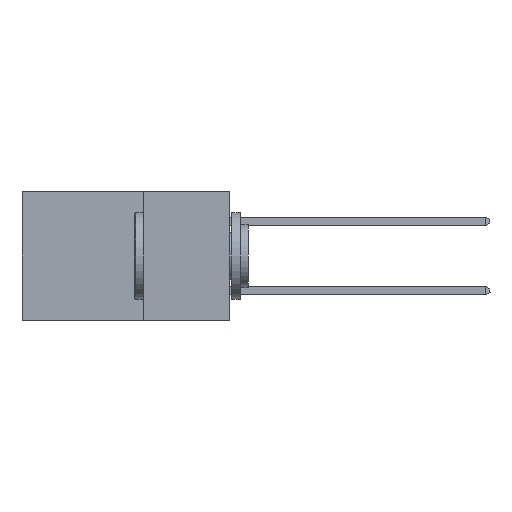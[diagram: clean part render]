
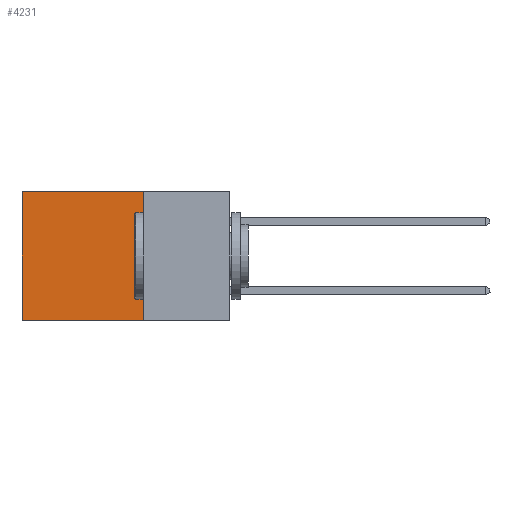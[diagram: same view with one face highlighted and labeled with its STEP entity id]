
A CAD part, left-side view. The second image highlights one B-rep face of the part: STEP entity #4231.
In plain terms, the highlighted planar face has unit normal (-1, 0, 0).
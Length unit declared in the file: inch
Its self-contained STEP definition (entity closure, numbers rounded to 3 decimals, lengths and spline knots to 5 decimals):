
#115 = ORIENTED_EDGE ( 'NONE', *, *, #20439, .F. ) ;
#172 = EDGE_CURVE ( 'NONE', #22856, #275, #1606, .T. ) ;
#275 = VERTEX_POINT ( 'NONE', #14383 ) ;
#527 = DIRECTION ( 'NONE',  ( 1., 0., 0. ) ) ;
#530 = PLANE ( 'NONE',  #2457 ) ;
#650 = DIRECTION ( 'NONE',  ( 0., 0., -1. ) ) ;
#1184 = DIRECTION ( 'NONE',  ( 0., 0., -1. ) ) ;
#1248 = VERTEX_POINT ( 'NONE', #6865 ) ;
#1606 = LINE ( 'NONE', #5514, #10733 ) ;
#2457 = AXIS2_PLACEMENT_3D ( 'NONE', #7439, #527, #16551 ) ;
#3480 = VECTOR ( 'NONE', #650, 39.37008 ) ;
#4231 = ADVANCED_FACE ( 'NONE', ( #7387 ), #530, .F. ) ;
#5514 = CARTESIAN_POINT ( 'NONE',  ( 0.298, 0.25, 0. ) ) ;
#5868 = DIRECTION ( 'NONE',  ( 0., 1., 0. ) ) ;
#6865 = CARTESIAN_POINT ( 'NONE',  ( 0.298, 0.25, -0.37 ) ) ;
#7387 = FACE_OUTER_BOUND ( 'NONE', #10016, .T. ) ;
#7439 = CARTESIAN_POINT ( 'NONE',  ( 0.298, 0.25, 0. ) ) ;
#7745 = LINE ( 'NONE', #8923, #17954 ) ;
#7750 = VECTOR ( 'NONE', #23144, 39.37008 ) ;
#7885 = CARTESIAN_POINT ( 'NONE',  ( 0.298, 0.25, -0.37 ) ) ;
#8923 = CARTESIAN_POINT ( 'NONE',  ( 0.298, 0.6, 0. ) ) ;
#8965 = LINE ( 'NONE', #7885, #7750 ) ;
#9561 = ORIENTED_EDGE ( 'NONE', *, *, #19912, .F. ) ;
#10016 = EDGE_LOOP ( 'NONE', ( #18781, #115, #9561, #10833 ) ) ;
#10733 = VECTOR ( 'NONE', #5868, 39.37008 ) ;
#10833 = ORIENTED_EDGE ( 'NONE', *, *, #172, .T. ) ;
#14383 = CARTESIAN_POINT ( 'NONE',  ( 0.298, 0.6, 0. ) ) ;
#16551 = DIRECTION ( 'NONE',  ( 0., 0., -1. ) ) ;
#16861 = CARTESIAN_POINT ( 'NONE',  ( 0.298, 0.25, 0. ) ) ;
#17954 = VECTOR ( 'NONE', #1184, 39.37008 ) ;
#18781 = ORIENTED_EDGE ( 'NONE', *, *, #19732, .T. ) ;
#19732 = EDGE_CURVE ( 'NONE', #275, #21724, #7745, .T. ) ;
#19879 = CARTESIAN_POINT ( 'NONE',  ( 0.298, 0.25, 0. ) ) ;
#19912 = EDGE_CURVE ( 'NONE', #22856, #1248, #24450, .T. ) ;
#20439 = EDGE_CURVE ( 'NONE', #1248, #21724, #8965, .T. ) ;
#21036 = CARTESIAN_POINT ( 'NONE',  ( 0.298, 0.6, -0.37 ) ) ;
#21724 = VERTEX_POINT ( 'NONE', #21036 ) ;
#22856 = VERTEX_POINT ( 'NONE', #16861 ) ;
#23144 = DIRECTION ( 'NONE',  ( 0., 1., 0. ) ) ;
#24450 = LINE ( 'NONE', #19879, #3480 ) ;
